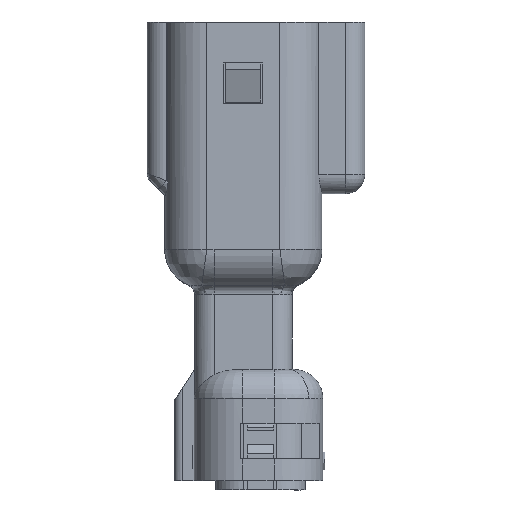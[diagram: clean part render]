
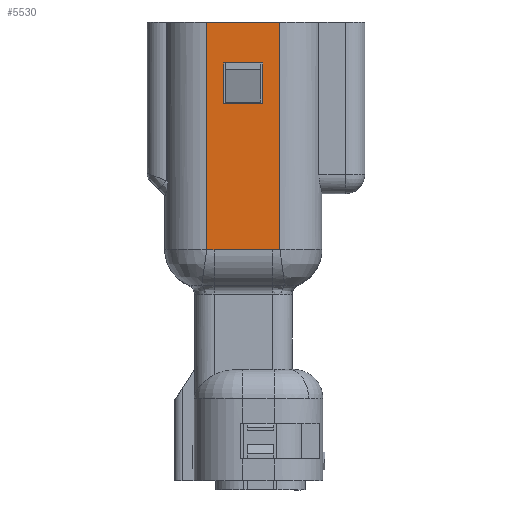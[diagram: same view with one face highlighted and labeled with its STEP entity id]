
A CAD part, left-side view. The second image highlights one B-rep face of the part: STEP entity #5530.
In plain terms, the highlighted planar face has unit normal (-1, 0, 0).
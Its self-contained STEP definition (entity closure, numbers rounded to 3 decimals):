
#87 = CARTESIAN_POINT ( 'NONE',  ( -4.65, 13.6, 1.875 ) ) ;
#127 = ORIENTED_EDGE ( 'NONE', *, *, #9791, .T. ) ;
#211 = EDGE_LOOP ( 'NONE', ( #24970, #7163, #24358, #20732, #661, #8835 ) ) ;
#530 = VERTEX_POINT ( 'NONE', #19319 ) ;
#622 = EDGE_CURVE ( 'NONE', #21532, #530, #14720, .T. ) ;
#634 = VERTEX_POINT ( 'NONE', #28587 ) ;
#658 = CARTESIAN_POINT ( 'NONE',  ( -4.65, 1.923, 1.5 ) ) ;
#661 = ORIENTED_EDGE ( 'NONE', *, *, #29373, .F. ) ;
#1009 = CARTESIAN_POINT ( 'NONE',  ( -4.65, 1.957, -1.875 ) ) ;
#1241 = CARTESIAN_POINT ( 'NONE',  ( -4.65, 1.948, 1.815 ) ) ;
#1667 = VERTEX_POINT ( 'NONE', #15458 ) ;
#2233 = DIRECTION ( 'NONE',  ( 0., 1., 0. ) ) ;
#3115 = VECTOR ( 'NONE', #2233, 1000. ) ;
#3296 =( BOUNDED_CURVE ( )  B_SPLINE_CURVE ( 3, ( #12549, #10770, #1241, #5849, #17056, #12708, #19263, #28678 ),
 .UNSPECIFIED., .F., .F. ) 
 B_SPLINE_CURVE_WITH_KNOTS ( ( 4, 1, 1, 1, 1, 4 ),
 ( 0., 0.096, 0.309, 0.53, 0.762, 1. ),
 .UNSPECIFIED. ) 
 CURVE ( )  GEOMETRIC_REPRESENTATION_ITEM ( )  RATIONAL_B_SPLINE_CURVE ( ( 1.097, 1.097, 1.097, 1.097, 1.097, 1.097, 1.097, 1.097 ) ) 
 REPRESENTATION_ITEM ( '' )  );
#3806 = LINE ( 'NONE', #8415, #29003 ) ;
#3948 = PLANE ( 'NONE',  #18501 ) ;
#3959 = CARTESIAN_POINT ( 'NONE',  ( -4.65, 9.4, -1. ) ) ;
#4001 = LINE ( 'NONE', #28622, #18281 ) ;
#4246 = DIRECTION ( 'NONE',  ( -1., 0., 0. ) ) ;
#4319 = LINE ( 'NONE', #22637, #3115 ) ;
#4357 = EDGE_CURVE ( 'NONE', #20917, #634, #3806, .T. ) ;
#4675 = CARTESIAN_POINT ( 'NONE',  ( -4.65, 13.6, -1.875 ) ) ;
#5269 = VECTOR ( 'NONE', #11540, 1000. ) ;
#5451 = CARTESIAN_POINT ( 'NONE',  ( -4.65, 1.948, -1.808 ) ) ;
#5530 = ADVANCED_FACE ( 'NONE', ( #10515, #6187 ), #3948, .T. ) ;
#5675 = EDGE_CURVE ( 'NONE', #25413, #12280, #11395, .T. ) ;
#5849 = CARTESIAN_POINT ( 'NONE',  ( -4.65, 1.939, 1.742 ) ) ;
#6187 = FACE_OUTER_BOUND ( 'NONE', #211, .T. ) ;
#6223 = CARTESIAN_POINT ( 'NONE',  ( -4.65, 9.4, 1. ) ) ;
#6302 = ORIENTED_EDGE ( 'NONE', *, *, #15501, .T. ) ;
#7163 = ORIENTED_EDGE ( 'NONE', *, *, #20655, .F. ) ;
#7704 = CARTESIAN_POINT ( 'NONE',  ( -4.65, 1.923, -1.526 ) ) ;
#8415 = CARTESIAN_POINT ( 'NONE',  ( -4.65, 11.5, -1. ) ) ;
#8835 = ORIENTED_EDGE ( 'NONE', *, *, #24398, .F. ) ;
#9083 = CARTESIAN_POINT ( 'NONE',  ( -4.65, 1.923, -1.5 ) ) ;
#9791 = EDGE_CURVE ( 'NONE', #21931, #29136, #29338, .T. ) ;
#10515 = FACE_BOUND ( 'NONE', #26195, .T. ) ;
#10770 = CARTESIAN_POINT ( 'NONE',  ( -4.65, 1.955, 1.861 ) ) ;
#11395 = LINE ( 'NONE', #27219, #5269 ) ;
#11540 = DIRECTION ( 'NONE',  ( 0., 1., 0. ) ) ;
#12280 = VERTEX_POINT ( 'NONE', #87 ) ;
#12314 = CARTESIAN_POINT ( 'NONE',  ( -4.65, 1.954, -1.857 ) ) ;
#12549 = CARTESIAN_POINT ( 'NONE',  ( -4.65, 1.957, 1.875 ) ) ;
#12685 = VERTEX_POINT ( 'NONE', #21048 ) ;
#12708 = CARTESIAN_POINT ( 'NONE',  ( -4.65, 1.924, 1.579 ) ) ;
#12905 = DIRECTION ( 'NONE',  ( 0., 0., 1. ) ) ;
#13378 = DIRECTION ( 'NONE',  ( 0., 1., 0. ) ) ;
#13787 = CARTESIAN_POINT ( 'NONE',  ( -4.65, 1.957, 1.875 ) ) ;
#14282 = EDGE_CURVE ( 'NONE', #634, #21931, #4001, .T. ) ;
#14409 = CARTESIAN_POINT ( 'NONE',  ( -4.65, 1.923, -1.5 ) ) ;
#14554 = CARTESIAN_POINT ( 'NONE',  ( -4.65, 1.924, -1.576 ) ) ;
#14720 =( BOUNDED_CURVE ( )  B_SPLINE_CURVE ( 3, ( #14409, #7704, #14554, #16806, #25899, #5451, #12314, #1009 ),
 .UNSPECIFIED., .F., .F. ) 
 B_SPLINE_CURVE_WITH_KNOTS ( ( 4, 1, 1, 1, 1, 4 ),
 ( 0., 0.231, 0.456, 0.67, 0.878, 1. ),
 .UNSPECIFIED. ) 
 CURVE ( )  GEOMETRIC_REPRESENTATION_ITEM ( )  RATIONAL_B_SPLINE_CURVE ( ( 1.097, 1.097, 1.097, 1.097, 1.097, 1.097, 1.097, 1.097 ) ) 
 REPRESENTATION_ITEM ( '' )  );
#15458 = CARTESIAN_POINT ( 'NONE',  ( -4.65, 13.6, -1.875 ) ) ;
#15501 = EDGE_CURVE ( 'NONE', #29136, #20917, #4319, .T. ) ;
#15757 = EDGE_CURVE ( 'NONE', #530, #1667, #20230, .T. ) ;
#16806 = CARTESIAN_POINT ( 'NONE',  ( -4.65, 1.93, -1.654 ) ) ;
#17056 = CARTESIAN_POINT ( 'NONE',  ( -4.65, 1.93, 1.659 ) ) ;
#17375 = CARTESIAN_POINT ( 'NONE',  ( -4.65, 0., -1.875 ) ) ;
#17480 = VECTOR ( 'NONE', #25308, 1000. ) ;
#18281 = VECTOR ( 'NONE', #26831, 1000. ) ;
#18501 = AXIS2_PLACEMENT_3D ( 'NONE', #17375, #4246, #28850 ) ;
#19263 = CARTESIAN_POINT ( 'NONE',  ( -4.65, 1.923, 1.527 ) ) ;
#19319 = CARTESIAN_POINT ( 'NONE',  ( -4.65, 1.957, -1.875 ) ) ;
#20230 = LINE ( 'NONE', #29049, #27459 ) ;
#20655 = EDGE_CURVE ( 'NONE', #1667, #12280, #27652, .T. ) ;
#20732 = ORIENTED_EDGE ( 'NONE', *, *, #622, .F. ) ;
#20917 = VERTEX_POINT ( 'NONE', #25982 ) ;
#20966 = VECTOR ( 'NONE', #26005, 1000. ) ;
#21048 = CARTESIAN_POINT ( 'NONE',  ( -4.65, 1.923, 1.5 ) ) ;
#21532 = VERTEX_POINT ( 'NONE', #9083 ) ;
#21931 = VERTEX_POINT ( 'NONE', #6223 ) ;
#21976 = ORIENTED_EDGE ( 'NONE', *, *, #14282, .T. ) ;
#22637 = CARTESIAN_POINT ( 'NONE',  ( -4.65, 9.4, -1. ) ) ;
#22890 = VECTOR ( 'NONE', #27212, 1000. ) ;
#23071 = ORIENTED_EDGE ( 'NONE', *, *, #4357, .T. ) ;
#24358 = ORIENTED_EDGE ( 'NONE', *, *, #15757, .F. ) ;
#24398 = EDGE_CURVE ( 'NONE', #25413, #12685, #3296, .T. ) ;
#24970 = ORIENTED_EDGE ( 'NONE', *, *, #5675, .T. ) ;
#25308 = DIRECTION ( 'NONE',  ( 0., 0., -1. ) ) ;
#25413 = VERTEX_POINT ( 'NONE', #13787 ) ;
#25415 = LINE ( 'NONE', #658, #20966 ) ;
#25899 = CARTESIAN_POINT ( 'NONE',  ( -4.65, 1.938, -1.734 ) ) ;
#25982 = CARTESIAN_POINT ( 'NONE',  ( -4.65, 11.5, -1. ) ) ;
#26005 = DIRECTION ( 'NONE',  ( 0., 0., -1. ) ) ;
#26195 = EDGE_LOOP ( 'NONE', ( #127, #6302, #23071, #21976 ) ) ;
#26831 = DIRECTION ( 'NONE',  ( 0., -1., 0. ) ) ;
#27212 = DIRECTION ( 'NONE',  ( 0., 0., 1. ) ) ;
#27219 = CARTESIAN_POINT ( 'NONE',  ( -4.65, 1.957, 1.875 ) ) ;
#27459 = VECTOR ( 'NONE', #13378, 1000. ) ;
#27559 = CARTESIAN_POINT ( 'NONE',  ( -4.65, 9.4, 1. ) ) ;
#27652 = LINE ( 'NONE', #4675, #22890 ) ;
#28587 = CARTESIAN_POINT ( 'NONE',  ( -4.65, 11.5, 1. ) ) ;
#28622 = CARTESIAN_POINT ( 'NONE',  ( -4.65, 11.5, 1. ) ) ;
#28678 = CARTESIAN_POINT ( 'NONE',  ( -4.65, 1.923, 1.5 ) ) ;
#28850 = DIRECTION ( 'NONE',  ( 0., 0., 1. ) ) ;
#29003 = VECTOR ( 'NONE', #12905, 1000. ) ;
#29049 = CARTESIAN_POINT ( 'NONE',  ( -4.65, 1.957, -1.875 ) ) ;
#29136 = VERTEX_POINT ( 'NONE', #3959 ) ;
#29338 = LINE ( 'NONE', #27559, #17480 ) ;
#29373 = EDGE_CURVE ( 'NONE', #12685, #21532, #25415, .T. ) ;
